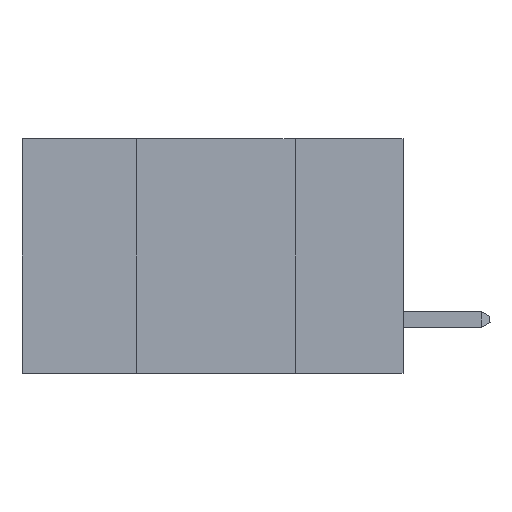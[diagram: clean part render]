
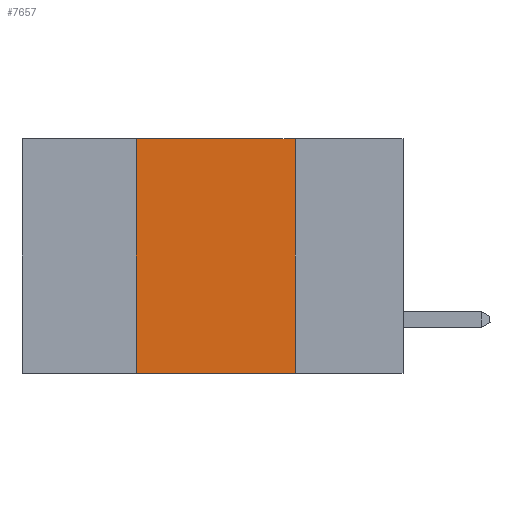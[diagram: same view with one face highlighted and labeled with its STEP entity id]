
A CAD part, left-side view. The second image highlights one B-rep face of the part: STEP entity #7657.
In plain terms, the highlighted planar face has unit normal (-1, 0, 0).
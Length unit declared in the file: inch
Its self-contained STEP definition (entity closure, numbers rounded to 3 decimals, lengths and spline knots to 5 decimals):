
#100 = DIRECTION ( 'NONE',  ( 0., -1., 0. ) ) ;
#1710 = FACE_OUTER_BOUND ( 'NONE', #15819, .T. ) ;
#1923 = EDGE_CURVE ( 'NONE', #7039, #5067, #10922, .T. ) ;
#1955 = LINE ( 'NONE', #10467, #18864 ) ;
#2369 = VECTOR ( 'NONE', #20937, 39.37008 ) ;
#2394 = ORIENTED_EDGE ( 'NONE', *, *, #13029, .F. ) ;
#2776 = CARTESIAN_POINT ( 'NONE',  ( 0., 0.6, 0. ) ) ;
#2837 = VERTEX_POINT ( 'NONE', #6453 ) ;
#3651 = CARTESIAN_POINT ( 'NONE',  ( 0., 0.17, -0.37 ) ) ;
#3810 = VECTOR ( 'NONE', #5073, 39.37008 ) ;
#3899 = DIRECTION ( 'NONE',  ( 1., 0., 0. ) ) ;
#5067 = VERTEX_POINT ( 'NONE', #6552 ) ;
#5073 = DIRECTION ( 'NONE',  ( 0., 0., -1. ) ) ;
#6453 = CARTESIAN_POINT ( 'NONE',  ( 0., 0.17, 0. ) ) ;
#6552 = CARTESIAN_POINT ( 'NONE',  ( 0., 0.42, 0. ) ) ;
#7039 = VERTEX_POINT ( 'NONE', #19032 ) ;
#7065 = DIRECTION ( 'NONE',  ( 0., -1., 0. ) ) ;
#7657 = ADVANCED_FACE ( 'NONE', ( #1710 ), #15690, .F. ) ;
#9757 = DIRECTION ( 'NONE',  ( 0., 0., -1. ) ) ;
#9843 = VERTEX_POINT ( 'NONE', #3651 ) ;
#10467 = CARTESIAN_POINT ( 'NONE',  ( 0., 0.6, -0.37 ) ) ;
#10901 = ORIENTED_EDGE ( 'NONE', *, *, #21650, .T. ) ;
#10922 = LINE ( 'NONE', #12134, #2369 ) ;
#12098 = CARTESIAN_POINT ( 'NONE',  ( 0., 0.6, 0. ) ) ;
#12134 = CARTESIAN_POINT ( 'NONE',  ( 0., 0.42, 0. ) ) ;
#13013 = ORIENTED_EDGE ( 'NONE', *, *, #1923, .F. ) ;
#13029 = EDGE_CURVE ( 'NONE', #2837, #9843, #21674, .T. ) ;
#13404 = VECTOR ( 'NONE', #100, 39.37008 ) ;
#13534 = CARTESIAN_POINT ( 'NONE',  ( 0., 0.17, 0. ) ) ;
#14467 = LINE ( 'NONE', #12098, #13404 ) ;
#14745 = AXIS2_PLACEMENT_3D ( 'NONE', #2776, #3899, #9757 ) ;
#15690 = PLANE ( 'NONE',  #14745 ) ;
#15819 = EDGE_LOOP ( 'NONE', ( #2394, #19471, #13013, #10901 ) ) ;
#16823 = EDGE_CURVE ( 'NONE', #5067, #2837, #14467, .T. ) ;
#18864 = VECTOR ( 'NONE', #7065, 39.37008 ) ;
#19032 = CARTESIAN_POINT ( 'NONE',  ( 0., 0.42, -0.37 ) ) ;
#19471 = ORIENTED_EDGE ( 'NONE', *, *, #16823, .F. ) ;
#20937 = DIRECTION ( 'NONE',  ( 0., 0., 1. ) ) ;
#21650 = EDGE_CURVE ( 'NONE', #7039, #9843, #1955, .T. ) ;
#21674 = LINE ( 'NONE', #13534, #3810 ) ;
